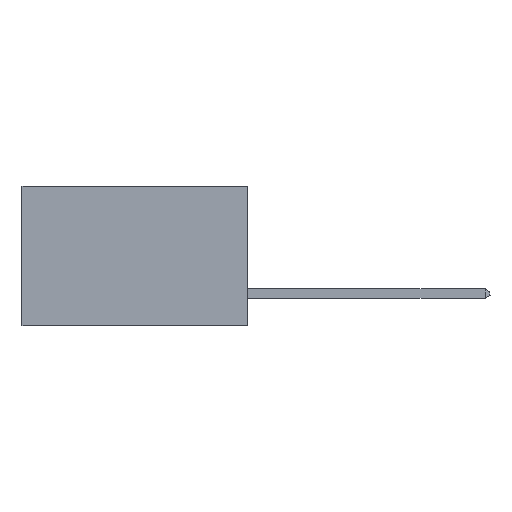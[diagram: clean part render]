
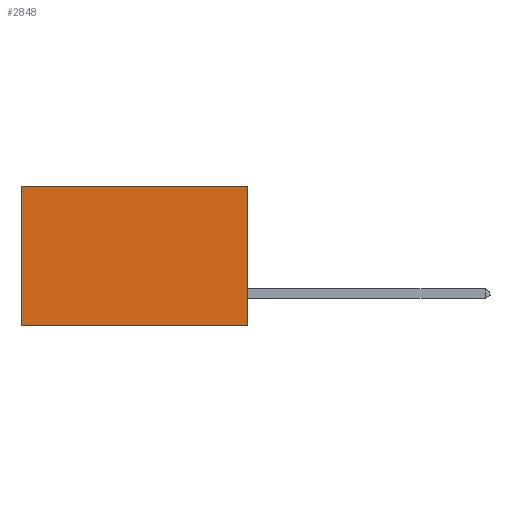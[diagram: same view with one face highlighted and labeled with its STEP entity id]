
A CAD part, left-side view. The second image highlights one B-rep face of the part: STEP entity #2848.
In plain terms, the highlighted planar face has unit normal (-1, 0, 0).
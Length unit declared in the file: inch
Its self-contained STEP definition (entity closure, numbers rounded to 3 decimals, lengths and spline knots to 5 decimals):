
#338 = VERTEX_POINT ( 'NONE', #812 ) ;
#812 = CARTESIAN_POINT ( 'NONE',  ( 0.298, 0., 0. ) ) ;
#1396 = CARTESIAN_POINT ( 'NONE',  ( 0.298, 0., 0. ) ) ;
#1568 = VERTEX_POINT ( 'NONE', #7066 ) ;
#1671 = CARTESIAN_POINT ( 'NONE',  ( 0.298, 0., -0.37 ) ) ;
#1720 = LINE ( 'NONE', #3664, #2403 ) ;
#2103 = VERTEX_POINT ( 'NONE', #8041 ) ;
#2113 = EDGE_LOOP ( 'NONE', ( #6567, #7659, #3520, #5999 ) ) ;
#2403 = VECTOR ( 'NONE', #4194, 39.37008 ) ;
#2478 = CARTESIAN_POINT ( 'NONE',  ( 0.298, 0.6, 0. ) ) ;
#2547 = CARTESIAN_POINT ( 'NONE',  ( 0.298, 0., 0. ) ) ;
#2816 = EDGE_CURVE ( 'NONE', #1568, #2103, #7700, .T. ) ;
#2848 = ADVANCED_FACE ( 'NONE', ( #6098 ), #6179, .F. ) ;
#3125 = EDGE_CURVE ( 'NONE', #338, #4752, #9314, .T. ) ;
#3307 = EDGE_CURVE ( 'NONE', #4752, #2103, #6920, .T. ) ;
#3461 = VECTOR ( 'NONE', #6760, 39.37008 ) ;
#3520 = ORIENTED_EDGE ( 'NONE', *, *, #3125, .F. ) ;
#3664 = CARTESIAN_POINT ( 'NONE',  ( 0.298, 0., 0. ) ) ;
#4022 = EDGE_CURVE ( 'NONE', #338, #1568, #1720, .T. ) ;
#4194 = DIRECTION ( 'NONE',  ( 0., 1., 0. ) ) ;
#4752 = VERTEX_POINT ( 'NONE', #7699 ) ;
#5066 = VECTOR ( 'NONE', #9421, 39.37008 ) ;
#5999 = ORIENTED_EDGE ( 'NONE', *, *, #4022, .T. ) ;
#6098 = FACE_OUTER_BOUND ( 'NONE', #2113, .T. ) ;
#6179 = PLANE ( 'NONE',  #8393 ) ;
#6567 = ORIENTED_EDGE ( 'NONE', *, *, #2816, .T. ) ;
#6760 = DIRECTION ( 'NONE',  ( 0., 1., 0. ) ) ;
#6920 = LINE ( 'NONE', #1671, #3461 ) ;
#7066 = CARTESIAN_POINT ( 'NONE',  ( 0.298, 0.6, 0. ) ) ;
#7648 = DIRECTION ( 'NONE',  ( 1., 0., 0. ) ) ;
#7659 = ORIENTED_EDGE ( 'NONE', *, *, #3307, .F. ) ;
#7699 = CARTESIAN_POINT ( 'NONE',  ( 0.298, 0., -0.37 ) ) ;
#7700 = LINE ( 'NONE', #2478, #9084 ) ;
#8041 = CARTESIAN_POINT ( 'NONE',  ( 0.298, 0.6, -0.37 ) ) ;
#8339 = DIRECTION ( 'NONE',  ( 0., 0., -1. ) ) ;
#8393 = AXIS2_PLACEMENT_3D ( 'NONE', #2547, #7648, #9104 ) ;
#9084 = VECTOR ( 'NONE', #8339, 39.37008 ) ;
#9104 = DIRECTION ( 'NONE',  ( 0., 0., -1. ) ) ;
#9314 = LINE ( 'NONE', #1396, #5066 ) ;
#9421 = DIRECTION ( 'NONE',  ( 0., 0., -1. ) ) ;
